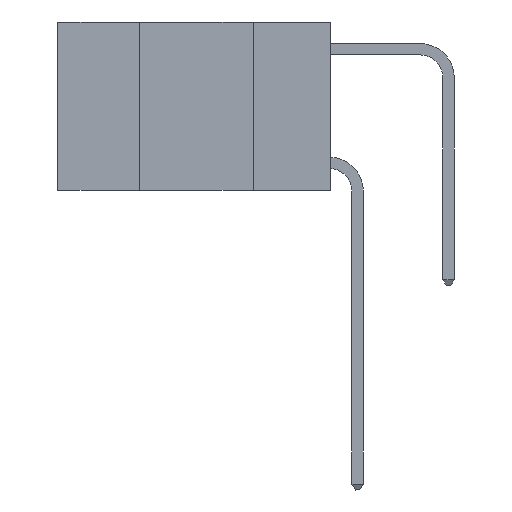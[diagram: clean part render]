
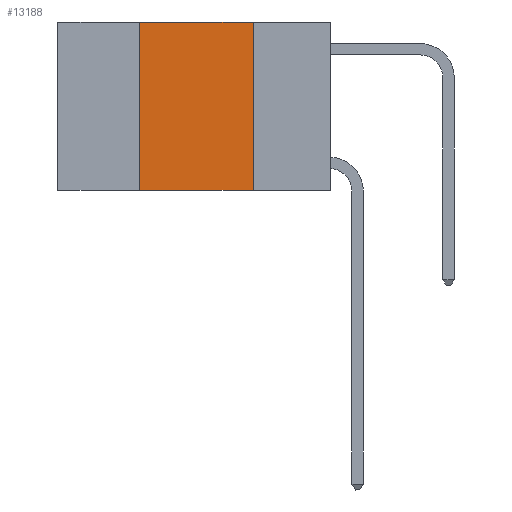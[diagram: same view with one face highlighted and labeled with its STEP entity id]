
A CAD part, left-side view. The second image highlights one B-rep face of the part: STEP entity #13188.
In plain terms, the highlighted planar face has unit normal (-1, 0, 0).
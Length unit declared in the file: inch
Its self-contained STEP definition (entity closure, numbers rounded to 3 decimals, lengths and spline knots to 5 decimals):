
#49 = LINE ( 'NONE', #7432, #16190 ) ;
#187 = ORIENTED_EDGE ( 'NONE', *, *, #14836, .F. ) ;
#2139 = EDGE_CURVE ( 'NONE', #4411, #9329, #49, .T. ) ;
#3515 = CARTESIAN_POINT ( 'NONE',  ( 0., 0.42, 0. ) ) ;
#4217 = VECTOR ( 'NONE', #19162, 39.37008 ) ;
#4240 = CARTESIAN_POINT ( 'NONE',  ( 0., 0.42, -0.37 ) ) ;
#4411 = VERTEX_POINT ( 'NONE', #19378 ) ;
#4786 = LINE ( 'NONE', #3515, #17120 ) ;
#5163 = AXIS2_PLACEMENT_3D ( 'NONE', #10598, #15121, #13540 ) ;
#6471 = PLANE ( 'NONE',  #5163 ) ;
#7432 = CARTESIAN_POINT ( 'NONE',  ( 0., 0.17, 0. ) ) ;
#7514 = EDGE_LOOP ( 'NONE', ( #12689, #9274, #187, #10847 ) ) ;
#7622 = DIRECTION ( 'NONE',  ( 0., 0., -1. ) ) ;
#8407 = CARTESIAN_POINT ( 'NONE',  ( 0., 0.42, 0. ) ) ;
#9274 = ORIENTED_EDGE ( 'NONE', *, *, #14614, .F. ) ;
#9329 = VERTEX_POINT ( 'NONE', #15768 ) ;
#9478 = DIRECTION ( 'NONE',  ( 0., 0., 1. ) ) ;
#10598 = CARTESIAN_POINT ( 'NONE',  ( 0., 0.6, 0. ) ) ;
#10847 = ORIENTED_EDGE ( 'NONE', *, *, #11204, .T. ) ;
#11204 = EDGE_CURVE ( 'NONE', #13020, #9329, #14567, .T. ) ;
#12689 = ORIENTED_EDGE ( 'NONE', *, *, #2139, .F. ) ;
#12741 = DIRECTION ( 'NONE',  ( 0., -1., 0. ) ) ;
#13020 = VERTEX_POINT ( 'NONE', #4240 ) ;
#13188 = ADVANCED_FACE ( 'NONE', ( #16884 ), #6471, .F. ) ;
#13540 = DIRECTION ( 'NONE',  ( 0., 0., -1. ) ) ;
#14567 = LINE ( 'NONE', #17891, #4217 ) ;
#14614 = EDGE_CURVE ( 'NONE', #15944, #4411, #15693, .T. ) ;
#14836 = EDGE_CURVE ( 'NONE', #13020, #15944, #4786, .T. ) ;
#15121 = DIRECTION ( 'NONE',  ( 1., 0., 0. ) ) ;
#15693 = LINE ( 'NONE', #17360, #17436 ) ;
#15768 = CARTESIAN_POINT ( 'NONE',  ( 0., 0.17, -0.37 ) ) ;
#15944 = VERTEX_POINT ( 'NONE', #8407 ) ;
#16190 = VECTOR ( 'NONE', #7622, 39.37008 ) ;
#16884 = FACE_OUTER_BOUND ( 'NONE', #7514, .T. ) ;
#17120 = VECTOR ( 'NONE', #9478, 39.37008 ) ;
#17360 = CARTESIAN_POINT ( 'NONE',  ( 0., 0.6, 0. ) ) ;
#17436 = VECTOR ( 'NONE', #12741, 39.37008 ) ;
#17891 = CARTESIAN_POINT ( 'NONE',  ( 0., 0.6, -0.37 ) ) ;
#19162 = DIRECTION ( 'NONE',  ( 0., -1., 0. ) ) ;
#19378 = CARTESIAN_POINT ( 'NONE',  ( 0., 0.17, 0. ) ) ;
